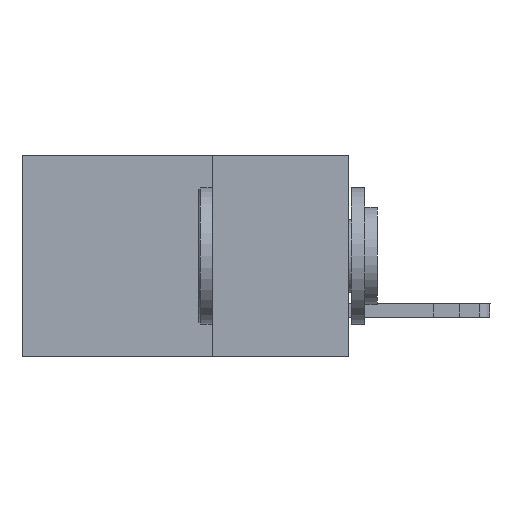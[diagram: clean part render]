
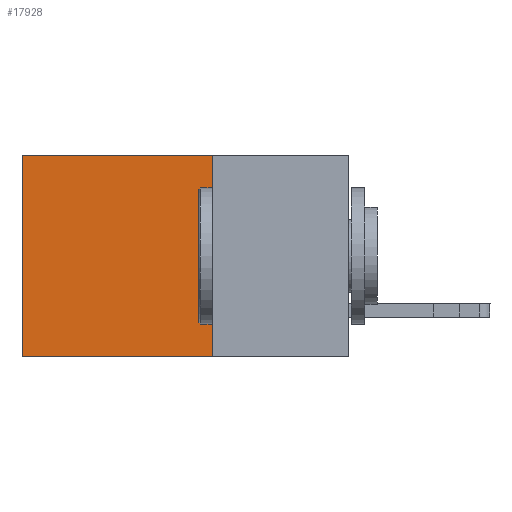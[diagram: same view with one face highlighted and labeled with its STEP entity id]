
A CAD part, left-side view. The second image highlights one B-rep face of the part: STEP entity #17928.
In plain terms, the highlighted planar face has unit normal (-1, 0, 0).
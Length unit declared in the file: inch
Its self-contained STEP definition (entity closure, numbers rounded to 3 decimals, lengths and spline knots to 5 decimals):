
#522 = CARTESIAN_POINT ( 'NONE',  ( 0.298, 0.6, -0.37 ) ) ;
#1828 = DIRECTION ( 'NONE',  ( 0., 0., -1. ) ) ;
#2818 = AXIS2_PLACEMENT_3D ( 'NONE', #8121, #20604, #13337 ) ;
#5450 = DIRECTION ( 'NONE',  ( 0., 0., -1. ) ) ;
#6047 = LINE ( 'NONE', #12538, #21178 ) ;
#6358 = VECTOR ( 'NONE', #11752, 39.37008 ) ;
#6380 = PLANE ( 'NONE',  #2818 ) ;
#6897 = VERTEX_POINT ( 'NONE', #21910 ) ;
#7508 = EDGE_CURVE ( 'NONE', #15531, #6897, #13095, .T. ) ;
#7747 = VERTEX_POINT ( 'NONE', #522 ) ;
#7789 = ORIENTED_EDGE ( 'NONE', *, *, #7508, .T. ) ;
#8121 = CARTESIAN_POINT ( 'NONE',  ( 0.298, 0.25, 0. ) ) ;
#8722 = LINE ( 'NONE', #10583, #17071 ) ;
#8742 = DIRECTION ( 'NONE',  ( 0., 1., 0. ) ) ;
#9724 = EDGE_CURVE ( 'NONE', #20416, #7747, #19448, .T. ) ;
#10583 = CARTESIAN_POINT ( 'NONE',  ( 0.298, 0.25, 0. ) ) ;
#10760 = CARTESIAN_POINT ( 'NONE',  ( 0.298, 0.25, -0.37 ) ) ;
#10864 = CARTESIAN_POINT ( 'NONE',  ( 0.298, 0.25, -0.37 ) ) ;
#11480 = ORIENTED_EDGE ( 'NONE', *, *, #9724, .F. ) ;
#11752 = DIRECTION ( 'NONE',  ( 0., 1., 0. ) ) ;
#12501 = ORIENTED_EDGE ( 'NONE', *, *, #18829, .F. ) ;
#12538 = CARTESIAN_POINT ( 'NONE',  ( 0.298, 0.6, 0. ) ) ;
#13095 = LINE ( 'NONE', #18843, #6358 ) ;
#13337 = DIRECTION ( 'NONE',  ( 0., 0., -1. ) ) ;
#14404 = EDGE_CURVE ( 'NONE', #6897, #7747, #6047, .T. ) ;
#15138 = FACE_OUTER_BOUND ( 'NONE', #19531, .T. ) ;
#15531 = VERTEX_POINT ( 'NONE', #22996 ) ;
#17071 = VECTOR ( 'NONE', #5450, 39.37008 ) ;
#17928 = ADVANCED_FACE ( 'NONE', ( #15138 ), #6380, .F. ) ;
#18596 = VECTOR ( 'NONE', #8742, 39.37008 ) ;
#18829 = EDGE_CURVE ( 'NONE', #15531, #20416, #8722, .T. ) ;
#18843 = CARTESIAN_POINT ( 'NONE',  ( 0.298, 0.25, 0. ) ) ;
#19448 = LINE ( 'NONE', #10760, #18596 ) ;
#19531 = EDGE_LOOP ( 'NONE', ( #22297, #11480, #12501, #7789 ) ) ;
#20416 = VERTEX_POINT ( 'NONE', #10864 ) ;
#20604 = DIRECTION ( 'NONE',  ( 1., 0., 0. ) ) ;
#21178 = VECTOR ( 'NONE', #1828, 39.37008 ) ;
#21910 = CARTESIAN_POINT ( 'NONE',  ( 0.298, 0.6, 0. ) ) ;
#22297 = ORIENTED_EDGE ( 'NONE', *, *, #14404, .T. ) ;
#22996 = CARTESIAN_POINT ( 'NONE',  ( 0.298, 0.25, 0. ) ) ;
